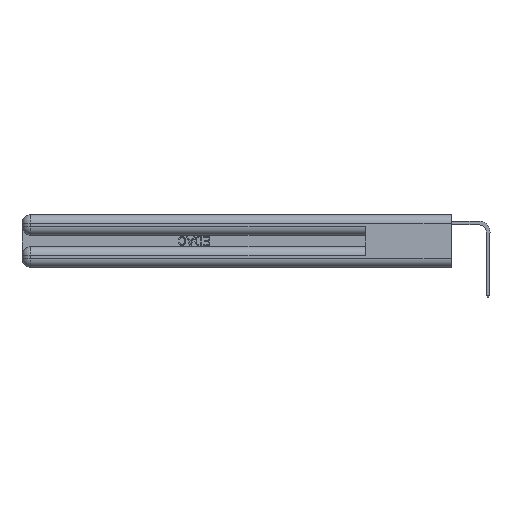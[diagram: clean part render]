
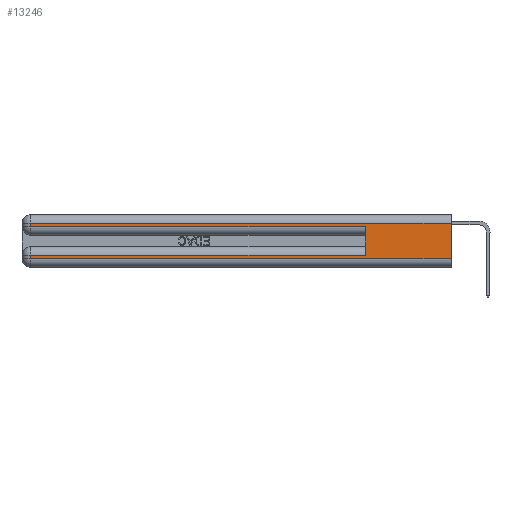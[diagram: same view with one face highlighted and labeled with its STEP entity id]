
A CAD part, left-side view. The second image highlights one B-rep face of the part: STEP entity #13246.
In plain terms, the highlighted planar face has unit normal (-1, 0, 0).
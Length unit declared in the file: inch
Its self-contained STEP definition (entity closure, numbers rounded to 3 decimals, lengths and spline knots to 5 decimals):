
#290 = CARTESIAN_POINT ( 'NONE',  ( 0., 0., 0.285 ) ) ;
#343 = VERTEX_POINT ( 'NONE', #5644 ) ;
#382 = LINE ( 'NONE', #23823, #11865 ) ;
#395 = CARTESIAN_POINT ( 'NONE',  ( 0., 0., 0.06 ) ) ;
#1055 = DIRECTION ( 'NONE',  ( 0., 0., -1. ) ) ;
#1326 = ORIENTED_EDGE ( 'NONE', *, *, #20319, .T. ) ;
#1327 = LINE ( 'NONE', #13273, #24083 ) ;
#1630 = CARTESIAN_POINT ( 'NONE',  ( 0., 0., 0.31 ) ) ;
#2873 = CARTESIAN_POINT ( 'NONE',  ( 0., 2.94, 0.31 ) ) ;
#2926 = EDGE_CURVE ( 'NONE', #11934, #14753, #10676, .T. ) ;
#3268 = CARTESIAN_POINT ( 'NONE',  ( 0., 0., 0.37 ) ) ;
#3826 = AXIS2_PLACEMENT_3D ( 'NONE', #3268, #14787, #1055 ) ;
#4168 = DIRECTION ( 'NONE',  ( 0., 1., 0. ) ) ;
#4471 = EDGE_CURVE ( 'NONE', #13850, #11934, #4599, .T. ) ;
#4599 = LINE ( 'NONE', #12963, #27949 ) ;
#5345 = VECTOR ( 'NONE', #25331, 39.37008 ) ;
#5644 = CARTESIAN_POINT ( 'NONE',  ( 0., 2.94, 0.085 ) ) ;
#5940 = VECTOR ( 'NONE', #11825, 39.37008 ) ;
#6012 = EDGE_CURVE ( 'NONE', #20012, #13850, #1327, .T. ) ;
#7543 = VECTOR ( 'NONE', #17963, 39.37008 ) ;
#8398 = DIRECTION ( 'NONE',  ( 0., 0., -1. ) ) ;
#8691 = VECTOR ( 'NONE', #17933, 39.37008 ) ;
#9014 = EDGE_CURVE ( 'NONE', #20012, #14581, #382, .T. ) ;
#9586 = EDGE_LOOP ( 'NONE', ( #28983, #26247, #11964, #27448, #15466, #9680, #19711, #1326 ) ) ;
#9680 = ORIENTED_EDGE ( 'NONE', *, *, #27782, .T. ) ;
#10129 = LINE ( 'NONE', #29056, #8691 ) ;
#10226 = VERTEX_POINT ( 'NONE', #19456 ) ;
#10676 = LINE ( 'NONE', #290, #5345 ) ;
#11825 = DIRECTION ( 'NONE',  ( 0., -1., 0. ) ) ;
#11865 = VECTOR ( 'NONE', #21685, 39.37008 ) ;
#11934 = VERTEX_POINT ( 'NONE', #20606 ) ;
#11964 = ORIENTED_EDGE ( 'NONE', *, *, #4471, .T. ) ;
#12963 = CARTESIAN_POINT ( 'NONE',  ( 0., 2.94, 0.37 ) ) ;
#13246 = ADVANCED_FACE ( 'NONE', ( #18713 ), #28216, .F. ) ;
#13273 = CARTESIAN_POINT ( 'NONE',  ( 0., 0., 0.31 ) ) ;
#13850 = VERTEX_POINT ( 'NONE', #2873 ) ;
#14581 = VERTEX_POINT ( 'NONE', #25847 ) ;
#14753 = VERTEX_POINT ( 'NONE', #26323 ) ;
#14787 = DIRECTION ( 'NONE',  ( 1., 0., 0. ) ) ;
#15113 = LINE ( 'NONE', #22392, #7543 ) ;
#15466 = ORIENTED_EDGE ( 'NONE', *, *, #29270, .F. ) ;
#17933 = DIRECTION ( 'NONE',  ( 0., 0., -1. ) ) ;
#17963 = DIRECTION ( 'NONE',  ( 0., 0., 1. ) ) ;
#18713 = FACE_OUTER_BOUND ( 'NONE', #9586, .T. ) ;
#19456 = CARTESIAN_POINT ( 'NONE',  ( 0., 0.6, 0.085 ) ) ;
#19498 = LINE ( 'NONE', #395, #5940 ) ;
#19711 = ORIENTED_EDGE ( 'NONE', *, *, #21823, .T. ) ;
#20012 = VERTEX_POINT ( 'NONE', #1630 ) ;
#20319 = EDGE_CURVE ( 'NONE', #28645, #14581, #19498, .T. ) ;
#20461 = CARTESIAN_POINT ( 'NONE',  ( 0., 2.94, 0.06 ) ) ;
#20606 = CARTESIAN_POINT ( 'NONE',  ( 0., 2.94, 0.285 ) ) ;
#21685 = DIRECTION ( 'NONE',  ( 0., 0., -1. ) ) ;
#21823 = EDGE_CURVE ( 'NONE', #343, #28645, #10129, .T. ) ;
#22392 = CARTESIAN_POINT ( 'NONE',  ( 0., 0.6, 0.145 ) ) ;
#23132 = DIRECTION ( 'NONE',  ( 0., 1., 0. ) ) ;
#23447 = VECTOR ( 'NONE', #23132, 39.37008 ) ;
#23727 = CARTESIAN_POINT ( 'NONE',  ( 0., 0., 0.085 ) ) ;
#23823 = CARTESIAN_POINT ( 'NONE',  ( 0., 0., 0.37 ) ) ;
#24083 = VECTOR ( 'NONE', #4168, 39.37008 ) ;
#25331 = DIRECTION ( 'NONE',  ( 0., -1., 0. ) ) ;
#25847 = CARTESIAN_POINT ( 'NONE',  ( 0., 0., 0.06 ) ) ;
#26247 = ORIENTED_EDGE ( 'NONE', *, *, #6012, .T. ) ;
#26323 = CARTESIAN_POINT ( 'NONE',  ( 0., 0.6, 0.285 ) ) ;
#27448 = ORIENTED_EDGE ( 'NONE', *, *, #2926, .T. ) ;
#27782 = EDGE_CURVE ( 'NONE', #10226, #343, #29359, .T. ) ;
#27949 = VECTOR ( 'NONE', #8398, 39.37008 ) ;
#28216 = PLANE ( 'NONE',  #3826 ) ;
#28645 = VERTEX_POINT ( 'NONE', #20461 ) ;
#28983 = ORIENTED_EDGE ( 'NONE', *, *, #9014, .F. ) ;
#29056 = CARTESIAN_POINT ( 'NONE',  ( 0., 2.94, 0.37 ) ) ;
#29270 = EDGE_CURVE ( 'NONE', #10226, #14753, #15113, .T. ) ;
#29359 = LINE ( 'NONE', #23727, #23447 ) ;
